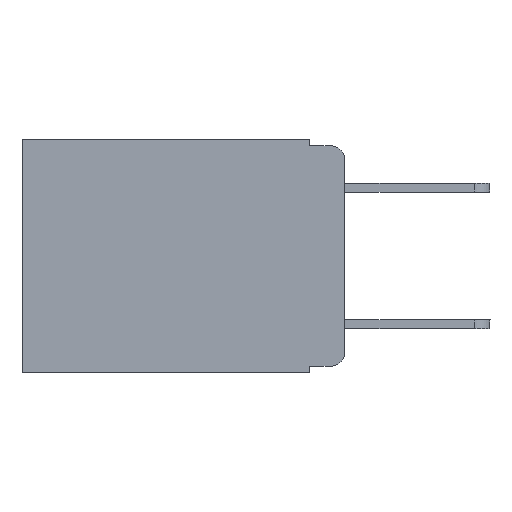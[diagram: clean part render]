
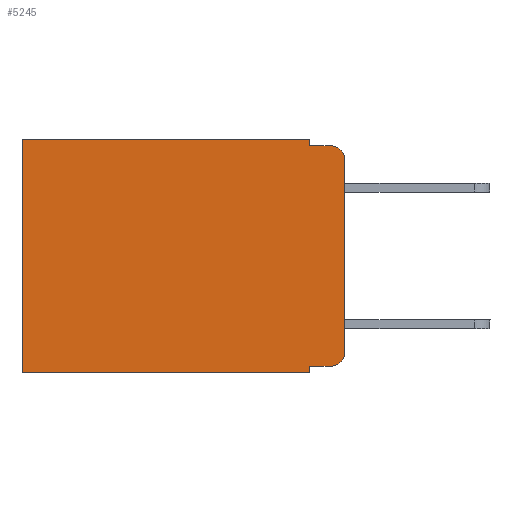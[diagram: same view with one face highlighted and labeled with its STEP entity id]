
A CAD part, left-side view. The second image highlights one B-rep face of the part: STEP entity #5245.
In plain terms, the highlighted planar face has unit normal (-1, 0, 0).
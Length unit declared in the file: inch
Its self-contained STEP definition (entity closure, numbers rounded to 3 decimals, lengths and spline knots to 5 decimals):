
#189 = VECTOR ( 'NONE', #3925, 39.37008 ) ;
#216 = VECTOR ( 'NONE', #8798, 39.37008 ) ;
#237 = LINE ( 'NONE', #11079, #4261 ) ;
#501 = ORIENTED_EDGE ( 'NONE', *, *, #4316, .T. ) ;
#751 = ORIENTED_EDGE ( 'NONE', *, *, #8589, .F. ) ;
#837 = LINE ( 'NONE', #1363, #3043 ) ;
#895 = DIRECTION ( 'NONE',  ( 0., -1., 0. ) ) ;
#934 = ORIENTED_EDGE ( 'NONE', *, *, #13113, .T. ) ;
#1251 = EDGE_CURVE ( 'NONE', #11882, #1684, #8090, .T. ) ;
#1363 = CARTESIAN_POINT ( 'NONE',  ( 0.298, 0.051, -0.333 ) ) ;
#1432 = LINE ( 'NONE', #3779, #12698 ) ;
#1587 = EDGE_CURVE ( 'NONE', #13438, #3666, #6720, .T. ) ;
#1684 = VERTEX_POINT ( 'NONE', #11636 ) ;
#1813 = CARTESIAN_POINT ( 'NONE',  ( 0.298, 0.051, -0.333 ) ) ;
#2185 = VERTEX_POINT ( 'NONE', #3330 ) ;
#2220 = EDGE_LOOP ( 'NONE', ( #6053, #3270, #9054, #11022, #8285, #934, #12867, #751, #501, #5931 ) ) ;
#2341 = DIRECTION ( 'NONE',  ( 0., 0., -1. ) ) ;
#2407 = DIRECTION ( 'NONE',  ( 0., -1., 0. ) ) ;
#2602 = EDGE_CURVE ( 'NONE', #13438, #3672, #237, .T. ) ;
#3043 = VECTOR ( 'NONE', #2407, 39.37008 ) ;
#3120 = VERTEX_POINT ( 'NONE', #9491 ) ;
#3270 = ORIENTED_EDGE ( 'NONE', *, *, #5971, .T. ) ;
#3273 = CARTESIAN_POINT ( 'NONE',  ( 0.298, 0.051, 0. ) ) ;
#3330 = CARTESIAN_POINT ( 'NONE',  ( 0.298, 0.02, -0.01 ) ) ;
#3331 = CARTESIAN_POINT ( 'NONE',  ( 0.298, 0.473, -0.343 ) ) ;
#3666 = VERTEX_POINT ( 'NONE', #12961 ) ;
#3672 = VERTEX_POINT ( 'NONE', #4199 ) ;
#3779 = CARTESIAN_POINT ( 'NONE',  ( 0.298, 0., -0.343 ) ) ;
#3874 = DIRECTION ( 'NONE',  ( -1., 0., 0. ) ) ;
#3925 = DIRECTION ( 'NONE',  ( 0., 0., -1. ) ) ;
#4141 = EDGE_CURVE ( 'NONE', #3666, #2185, #13630, .T. ) ;
#4199 = CARTESIAN_POINT ( 'NONE',  ( 0.298, 0.473, 0. ) ) ;
#4261 = VECTOR ( 'NONE', #4513, 39.37008 ) ;
#4316 = EDGE_CURVE ( 'NONE', #4986, #7035, #837, .T. ) ;
#4513 = DIRECTION ( 'NONE',  ( 0., 1., 0. ) ) ;
#4926 = DIRECTION ( 'NONE',  ( 0., 1., 0. ) ) ;
#4986 = VERTEX_POINT ( 'NONE', #1813 ) ;
#4987 = AXIS2_PLACEMENT_3D ( 'NONE', #7832, #12212, #13640 ) ;
#5175 = VECTOR ( 'NONE', #11395, 39.37008 ) ;
#5245 = ADVANCED_FACE ( 'NONE', ( #10668 ), #6833, .F. ) ;
#5392 = AXIS2_PLACEMENT_3D ( 'NONE', #5992, #3874, #11533 ) ;
#5621 = CARTESIAN_POINT ( 'NONE',  ( 0.298, 0., 0. ) ) ;
#5931 = ORIENTED_EDGE ( 'NONE', *, *, #9956, .T. ) ;
#5935 = EDGE_CURVE ( 'NONE', #3120, #8005, #1432, .T. ) ;
#5971 = EDGE_CURVE ( 'NONE', #11882, #2185, #6042, .T. ) ;
#5992 = CARTESIAN_POINT ( 'NONE',  ( 0.298, 0.02, -0.03 ) ) ;
#6042 = CIRCLE ( 'NONE', #5392, 0.02 ) ;
#6053 = ORIENTED_EDGE ( 'NONE', *, *, #1251, .F. ) ;
#6660 = CARTESIAN_POINT ( 'NONE',  ( 0.298, 0.051, 0. ) ) ;
#6691 = AXIS2_PLACEMENT_3D ( 'NONE', #5621, #7878, #2341 ) ;
#6720 = LINE ( 'NONE', #6958, #6894 ) ;
#6833 = PLANE ( 'NONE',  #6691 ) ;
#6894 = VECTOR ( 'NONE', #12005, 39.37008 ) ;
#6958 = CARTESIAN_POINT ( 'NONE',  ( 0.298, 0.051, 0. ) ) ;
#7035 = VERTEX_POINT ( 'NONE', #11701 ) ;
#7382 = CARTESIAN_POINT ( 'NONE',  ( 0.298, 0., -0.03 ) ) ;
#7832 = CARTESIAN_POINT ( 'NONE',  ( 0.298, 0.02, -0.313 ) ) ;
#7878 = DIRECTION ( 'NONE',  ( 1., 0., 0. ) ) ;
#8005 = VERTEX_POINT ( 'NONE', #3331 ) ;
#8090 = LINE ( 'NONE', #10214, #5175 ) ;
#8285 = ORIENTED_EDGE ( 'NONE', *, *, #2602, .T. ) ;
#8589 = EDGE_CURVE ( 'NONE', #4986, #3120, #13158, .T. ) ;
#8798 = DIRECTION ( 'NONE',  ( 0., 0., -1. ) ) ;
#9054 = ORIENTED_EDGE ( 'NONE', *, *, #4141, .F. ) ;
#9427 = CARTESIAN_POINT ( 'NONE',  ( 0.298, 0.051, -0.01 ) ) ;
#9479 = CARTESIAN_POINT ( 'NONE',  ( 0.298, 0.473, 0. ) ) ;
#9491 = CARTESIAN_POINT ( 'NONE',  ( 0.298, 0.051, -0.343 ) ) ;
#9956 = EDGE_CURVE ( 'NONE', #7035, #1684, #11401, .T. ) ;
#10040 = VECTOR ( 'NONE', #895, 39.37008 ) ;
#10214 = CARTESIAN_POINT ( 'NONE',  ( 0.298, 0., 0. ) ) ;
#10668 = FACE_OUTER_BOUND ( 'NONE', #2220, .T. ) ;
#11022 = ORIENTED_EDGE ( 'NONE', *, *, #1587, .F. ) ;
#11079 = CARTESIAN_POINT ( 'NONE',  ( 0.298, 0., 0. ) ) ;
#11395 = DIRECTION ( 'NONE',  ( 0., 0., -1. ) ) ;
#11401 = CIRCLE ( 'NONE', #4987, 0.02 ) ;
#11533 = DIRECTION ( 'NONE',  ( 0., 0., -1. ) ) ;
#11636 = CARTESIAN_POINT ( 'NONE',  ( 0.298, 0., -0.313 ) ) ;
#11701 = CARTESIAN_POINT ( 'NONE',  ( 0.298, 0.02, -0.333 ) ) ;
#11882 = VERTEX_POINT ( 'NONE', #7382 ) ;
#12005 = DIRECTION ( 'NONE',  ( 0., 0., -1. ) ) ;
#12212 = DIRECTION ( 'NONE',  ( -1., 0., 0. ) ) ;
#12451 = LINE ( 'NONE', #9479, #189 ) ;
#12698 = VECTOR ( 'NONE', #4926, 39.37008 ) ;
#12867 = ORIENTED_EDGE ( 'NONE', *, *, #5935, .F. ) ;
#12961 = CARTESIAN_POINT ( 'NONE',  ( 0.298, 0.051, -0.01 ) ) ;
#13113 = EDGE_CURVE ( 'NONE', #3672, #8005, #12451, .T. ) ;
#13158 = LINE ( 'NONE', #3273, #216 ) ;
#13438 = VERTEX_POINT ( 'NONE', #6660 ) ;
#13630 = LINE ( 'NONE', #9427, #10040 ) ;
#13640 = DIRECTION ( 'NONE',  ( 0., 0., -1. ) ) ;
